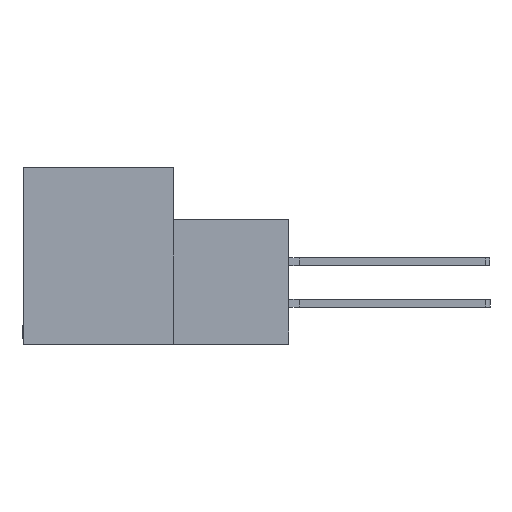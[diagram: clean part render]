
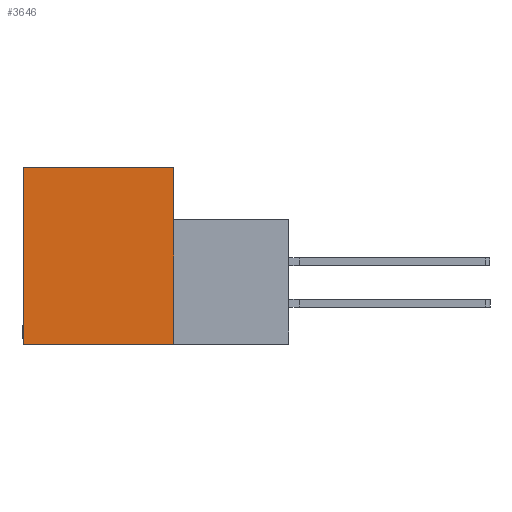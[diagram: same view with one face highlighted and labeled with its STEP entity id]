
A CAD part, left-side view. The second image highlights one B-rep face of the part: STEP entity #3646.
In plain terms, the highlighted planar face has unit normal (-1, 0, 0).
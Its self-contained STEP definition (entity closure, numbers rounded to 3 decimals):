
#1617 = VECTOR ( 'NONE', #26634, 1000. ) ;
#2504 = VECTOR ( 'NONE', #3730, 1000. ) ;
#2789 = CARTESIAN_POINT ( 'NONE',  ( 0., 11.506, -13.487 ) ) ;
#2952 = VERTEX_POINT ( 'NONE', #24404 ) ;
#3646 = ADVANCED_FACE ( 'NONE', ( #23616 ), #9068, .F. ) ;
#3730 = DIRECTION ( 'NONE',  ( 0., 1., 0. ) ) ;
#4401 = CARTESIAN_POINT ( 'NONE',  ( 0., 11.506, -13.487 ) ) ;
#4984 = CARTESIAN_POINT ( 'NONE',  ( 0., 0., 0. ) ) ;
#6077 = LINE ( 'NONE', #4401, #13718 ) ;
#6544 = EDGE_LOOP ( 'NONE', ( #14415, #21133, #28511, #32094 ) ) ;
#7548 = LINE ( 'NONE', #17701, #33193 ) ;
#9068 = PLANE ( 'NONE',  #10633 ) ;
#9191 = CARTESIAN_POINT ( 'NONE',  ( 0., 0., 0. ) ) ;
#9799 = DIRECTION ( 'NONE',  ( 0., -1., 0. ) ) ;
#9981 = EDGE_CURVE ( 'NONE', #24140, #32340, #15956, .T. ) ;
#10633 = AXIS2_PLACEMENT_3D ( 'NONE', #14174, #11541, #25524 ) ;
#11541 = DIRECTION ( 'NONE',  ( 1., 0., 0. ) ) ;
#13377 = CARTESIAN_POINT ( 'NONE',  ( 0., 0., -13.487 ) ) ;
#13718 = VECTOR ( 'NONE', #31297, 1000. ) ;
#14174 = CARTESIAN_POINT ( 'NONE',  ( 0., 0., 0. ) ) ;
#14415 = ORIENTED_EDGE ( 'NONE', *, *, #20514, .F. ) ;
#14477 = CARTESIAN_POINT ( 'NONE',  ( 0., -8.814, -13.487 ) ) ;
#15956 = LINE ( 'NONE', #4984, #1617 ) ;
#17495 = VERTEX_POINT ( 'NONE', #2789 ) ;
#17701 = CARTESIAN_POINT ( 'NONE',  ( 0., 11.506, 0. ) ) ;
#17807 = EDGE_CURVE ( 'NONE', #17495, #2952, #6077, .T. ) ;
#20514 = EDGE_CURVE ( 'NONE', #32340, #17495, #31088, .T. ) ;
#21133 = ORIENTED_EDGE ( 'NONE', *, *, #9981, .F. ) ;
#23616 = FACE_OUTER_BOUND ( 'NONE', #6544, .T. ) ;
#24140 = VERTEX_POINT ( 'NONE', #9191 ) ;
#24404 = CARTESIAN_POINT ( 'NONE',  ( 0., 11.506, 0. ) ) ;
#25524 = DIRECTION ( 'NONE',  ( 0., 0., -1. ) ) ;
#26329 = EDGE_CURVE ( 'NONE', #2952, #24140, #7548, .T. ) ;
#26634 = DIRECTION ( 'NONE',  ( 0., 0., -1. ) ) ;
#28511 = ORIENTED_EDGE ( 'NONE', *, *, #26329, .F. ) ;
#31088 = LINE ( 'NONE', #14477, #2504 ) ;
#31297 = DIRECTION ( 'NONE',  ( 0., 0., 1. ) ) ;
#32094 = ORIENTED_EDGE ( 'NONE', *, *, #17807, .F. ) ;
#32340 = VERTEX_POINT ( 'NONE', #13377 ) ;
#33193 = VECTOR ( 'NONE', #9799, 1000. ) ;
